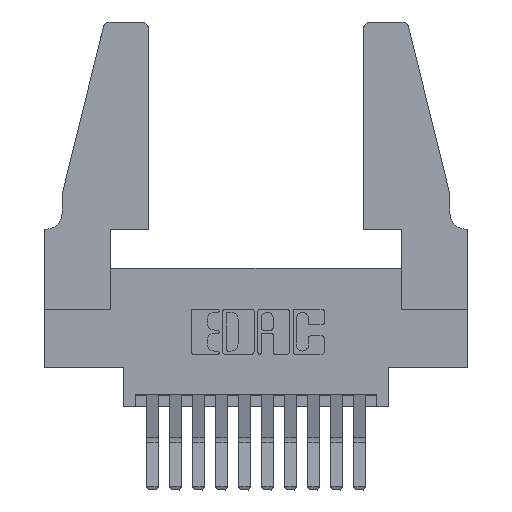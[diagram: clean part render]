
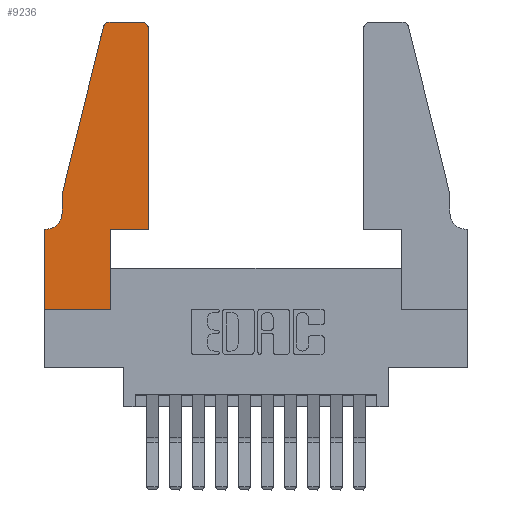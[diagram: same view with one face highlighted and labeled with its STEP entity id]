
A CAD part, top view. The second image highlights one B-rep face of the part: STEP entity #9236.
In plain terms, the highlighted planar face has unit normal (0, 0, 1).
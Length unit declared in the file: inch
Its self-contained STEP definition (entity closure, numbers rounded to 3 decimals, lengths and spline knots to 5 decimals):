
#285 = DIRECTION ( 'NONE',  ( 1., 0., 0. ) ) ;
#563 = ORIENTED_EDGE ( 'NONE', *, *, #11198, .T. ) ;
#652 = CARTESIAN_POINT ( 'NONE',  ( 0., 0.35, 0.37 ) ) ;
#1043 = DIRECTION ( 'NONE',  ( 0., 0., 1. ) ) ;
#1103 = FACE_OUTER_BOUND ( 'NONE', #12809, .T. ) ;
#1129 = VECTOR ( 'NONE', #285, 39.37008 ) ;
#1211 = ORIENTED_EDGE ( 'NONE', *, *, #1470, .T. ) ;
#1317 = VECTOR ( 'NONE', #10090, 39.37008 ) ;
#1470 = EDGE_CURVE ( 'NONE', #6767, #8577, #11215, .T. ) ;
#1591 = EDGE_CURVE ( 'NONE', #3368, #9420, #7156, .T. ) ;
#1692 = ORIENTED_EDGE ( 'NONE', *, *, #5337, .T. ) ;
#1732 = CIRCLE ( 'NONE', #6515, 0.07 ) ;
#1974 = VERTEX_POINT ( 'NONE', #2514 ) ;
#2128 = EDGE_CURVE ( 'NONE', #8577, #3014, #6428, .T. ) ;
#2145 = CARTESIAN_POINT ( 'NONE',  ( 0.0755, 0.5, 0.37 ) ) ;
#2202 = EDGE_CURVE ( 'NONE', #5900, #12764, #14290, .T. ) ;
#2514 = CARTESIAN_POINT ( 'NONE',  ( 0.4505, 1.22, 0.37 ) ) ;
#2961 = AXIS2_PLACEMENT_3D ( 'NONE', #8730, #13180, #6502 ) ;
#3014 = VERTEX_POINT ( 'NONE', #11787 ) ;
#3149 = ORIENTED_EDGE ( 'NONE', *, *, #2202, .T. ) ;
#3368 = VERTEX_POINT ( 'NONE', #9110 ) ;
#3476 = ORIENTED_EDGE ( 'NONE', *, *, #10547, .T. ) ;
#3880 = DIRECTION ( 'NONE',  ( 0., 0., -1. ) ) ;
#4280 = EDGE_CURVE ( 'NONE', #9322, #6767, #1732, .T. ) ;
#4417 = CARTESIAN_POINT ( 'NONE',  ( 0.284, 1.22, 0.37 ) ) ;
#4477 = CARTESIAN_POINT ( 'NONE',  ( 0., 0., 0.37 ) ) ;
#4518 = CARTESIAN_POINT ( 'NONE',  ( 0.2865, 0.35, 0.37 ) ) ;
#4560 = DIRECTION ( 'NONE',  ( 0., 1., 0. ) ) ;
#4735 = CARTESIAN_POINT ( 'NONE',  ( 0.2865, 0.35, 0.37 ) ) ;
#4739 = VECTOR ( 'NONE', #11247, 39.37008 ) ;
#5254 = LINE ( 'NONE', #13465, #14196 ) ;
#5280 = ORIENTED_EDGE ( 'NONE', *, *, #11864, .T. ) ;
#5337 = EDGE_CURVE ( 'NONE', #13673, #5796, #5254, .T. ) ;
#5399 = ORIENTED_EDGE ( 'NONE', *, *, #4280, .T. ) ;
#5407 = CARTESIAN_POINT ( 'NONE',  ( 0.0755, 0.35, 0.37 ) ) ;
#5426 = DIRECTION ( 'NONE',  ( -1., 0., 0. ) ) ;
#5470 = VECTOR ( 'NONE', #6786, 39.37008 ) ;
#5502 = CARTESIAN_POINT ( 'NONE',  ( 0.0755, 0.42, 0.37 ) ) ;
#5550 = DIRECTION ( 'NONE',  ( 1., 0., 0. ) ) ;
#5557 = CARTESIAN_POINT ( 'NONE',  ( 0.284, 1.25, 0.37 ) ) ;
#5796 = VERTEX_POINT ( 'NONE', #8850 ) ;
#5900 = VERTEX_POINT ( 'NONE', #9052 ) ;
#6232 = ORIENTED_EDGE ( 'NONE', *, *, #2128, .T. ) ;
#6428 = LINE ( 'NONE', #9781, #12030 ) ;
#6432 = ORIENTED_EDGE ( 'NONE', *, *, #8299, .T. ) ;
#6502 = DIRECTION ( 'NONE',  ( 1., 0., 0. ) ) ;
#6515 = AXIS2_PLACEMENT_3D ( 'NONE', #10662, #3880, #11765 ) ;
#6767 = VERTEX_POINT ( 'NONE', #14525 ) ;
#6785 = DIRECTION ( 'NONE',  ( -0.239, -0.971, 0. ) ) ;
#6786 = DIRECTION ( 'NONE',  ( 0., 1., 0. ) ) ;
#7156 = LINE ( 'NONE', #4735, #12731 ) ;
#7848 = CARTESIAN_POINT ( 'NONE',  ( 0.4205, 1.22, 0.37 ) ) ;
#8080 = EDGE_CURVE ( 'NONE', #5796, #9322, #13291, .T. ) ;
#8104 = LINE ( 'NONE', #4477, #4739 ) ;
#8105 = ORIENTED_EDGE ( 'NONE', *, *, #12783, .T. ) ;
#8299 = EDGE_CURVE ( 'NONE', #9420, #9775, #10190, .T. ) ;
#8367 = VECTOR ( 'NONE', #14010, 39.37008 ) ;
#8489 = LINE ( 'NONE', #13466, #5470 ) ;
#8569 = VECTOR ( 'NONE', #5426, 39.37008 ) ;
#8577 = VERTEX_POINT ( 'NONE', #652 ) ;
#8656 = AXIS2_PLACEMENT_3D ( 'NONE', #7848, #1043, #9000 ) ;
#8730 = CARTESIAN_POINT ( 'NONE',  ( 0., 0.35, 0.37 ) ) ;
#8850 = CARTESIAN_POINT ( 'NONE',  ( 0.0755, 0.5, 0.37 ) ) ;
#9000 = DIRECTION ( 'NONE',  ( 1., 0., 0. ) ) ;
#9052 = CARTESIAN_POINT ( 'NONE',  ( 0.4205, 1.25, 0.37 ) ) ;
#9110 = CARTESIAN_POINT ( 'NONE',  ( 0.2865, 0., 0.37 ) ) ;
#9216 = ORIENTED_EDGE ( 'NONE', *, *, #8080, .T. ) ;
#9236 = ADVANCED_FACE ( 'NONE', ( #1103 ), #12078, .T. ) ;
#9322 = VERTEX_POINT ( 'NONE', #5502 ) ;
#9420 = VERTEX_POINT ( 'NONE', #4518 ) ;
#9775 = VERTEX_POINT ( 'NONE', #11883 ) ;
#9781 = CARTESIAN_POINT ( 'NONE',  ( 0., 0., 0.37 ) ) ;
#9885 = DIRECTION ( 'NONE',  ( 0., -1., 0. ) ) ;
#10090 = DIRECTION ( 'NONE',  ( 0., -1., 0. ) ) ;
#10190 = LINE ( 'NONE', #13752, #1129 ) ;
#10361 = AXIS2_PLACEMENT_3D ( 'NONE', #4417, #12268, #5550 ) ;
#10547 = EDGE_CURVE ( 'NONE', #1974, #5900, #14097, .T. ) ;
#10662 = CARTESIAN_POINT ( 'NONE',  ( 0.0055, 0.42, 0.37 ) ) ;
#11198 = EDGE_CURVE ( 'NONE', #12764, #13673, #11334, .T. ) ;
#11215 = LINE ( 'NONE', #5407, #8569 ) ;
#11247 = DIRECTION ( 'NONE',  ( 1., 0., 0. ) ) ;
#11334 = CIRCLE ( 'NONE', #10361, 0.03 ) ;
#11765 = DIRECTION ( 'NONE',  ( -1., 0., 0. ) ) ;
#11787 = CARTESIAN_POINT ( 'NONE',  ( 0., 0., 0.37 ) ) ;
#11864 = EDGE_CURVE ( 'NONE', #9775, #1974, #8489, .T. ) ;
#11883 = CARTESIAN_POINT ( 'NONE',  ( 0.4505, 0.35, 0.37 ) ) ;
#12030 = VECTOR ( 'NONE', #9885, 39.37008 ) ;
#12078 = PLANE ( 'NONE',  #2961 ) ;
#12268 = DIRECTION ( 'NONE',  ( 0., 0., 1. ) ) ;
#12438 = CARTESIAN_POINT ( 'NONE',  ( 0.2605, 1.25, 0.37 ) ) ;
#12731 = VECTOR ( 'NONE', #4560, 39.37008 ) ;
#12764 = VERTEX_POINT ( 'NONE', #5557 ) ;
#12783 = EDGE_CURVE ( 'NONE', #3014, #3368, #8104, .T. ) ;
#12809 = EDGE_LOOP ( 'NONE', ( #3149, #563, #1692, #9216, #5399, #1211, #6232, #8105, #13203, #6432, #5280, #3476 ) ) ;
#13180 = DIRECTION ( 'NONE',  ( 0., 0., 1. ) ) ;
#13203 = ORIENTED_EDGE ( 'NONE', *, *, #1591, .T. ) ;
#13291 = LINE ( 'NONE', #2145, #1317 ) ;
#13465 = CARTESIAN_POINT ( 'NONE',  ( 0.0755, 0.5, 0.37 ) ) ;
#13466 = CARTESIAN_POINT ( 'NONE',  ( 0.4505, 0.35, 0.37 ) ) ;
#13673 = VERTEX_POINT ( 'NONE', #13761 ) ;
#13752 = CARTESIAN_POINT ( 'NONE',  ( 0.4505, 0.35, 0.37 ) ) ;
#13761 = CARTESIAN_POINT ( 'NONE',  ( 0.25487, 1.22718, 0.37 ) ) ;
#14010 = DIRECTION ( 'NONE',  ( -1., 0., 0. ) ) ;
#14097 = CIRCLE ( 'NONE', #8656, 0.03 ) ;
#14196 = VECTOR ( 'NONE', #6785, 39.37008 ) ;
#14290 = LINE ( 'NONE', #12438, #8367 ) ;
#14525 = CARTESIAN_POINT ( 'NONE',  ( 0.0055, 0.35, 0.37 ) ) ;
